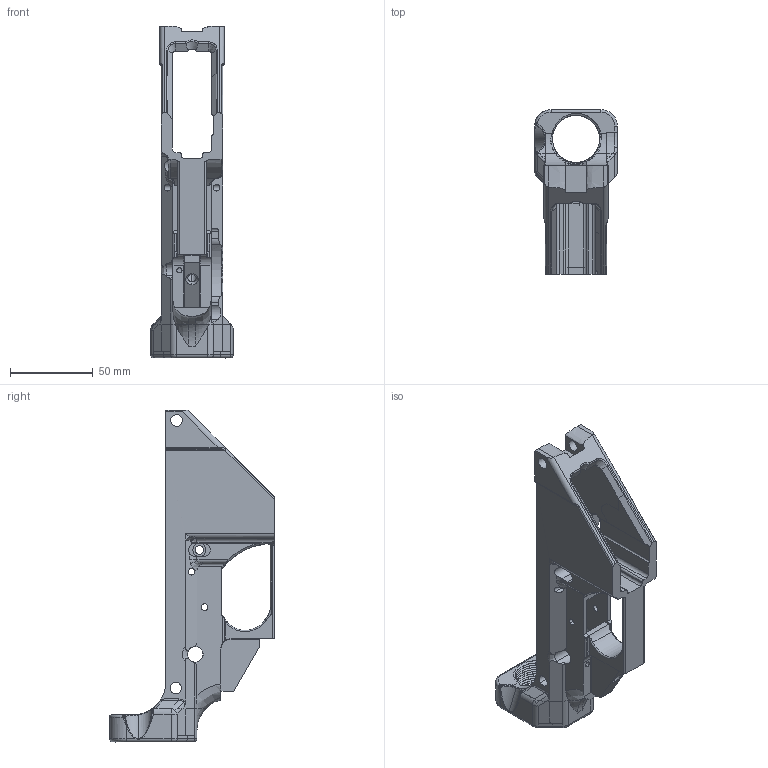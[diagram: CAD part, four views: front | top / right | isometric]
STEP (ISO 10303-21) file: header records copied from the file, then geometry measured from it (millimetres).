
FILE_DESCRIPTION (( 'STEP AP214' ), '1' );
FILE_NAME ('JT_Vanguard_Update FP.STEP', '2015-09-01T23:27:21', ( '' ), ( '' ), 'SwSTEP 2.0', 'SolidWorks 2015', '' );
FILE_SCHEMA (( 'AUTOMOTIVE_DESIGN' ));
Length unit declared in the file: millimetre
Products named in the file (1): JT_Vanguard_Update FP
Bounding box: 50 x 99.72 x 200.87 mm (x, y, z)
Volume: 160604.3 mm3; surface area: 59180.5 mm2
Topology: 2 solids, 2 shells, 600 faces, 1710 edges, 1095 vertices
Faces by surface type: cylinder 258, bspline 160, plane 154, torus 13, cone 12, sphere 3
Entity records: 37408 total; most frequent: CARTESIAN_POINT 23590, ORIENTED_EDGE 3400, DIRECTION 2209, EDGE_CURVE 1700, VERTEX_POINT 1095, AXIS2_PLACEMENT_3D 803, B_SPLINE_CURVE_WITH_KNOTS 640, EDGE_LOOP 629
